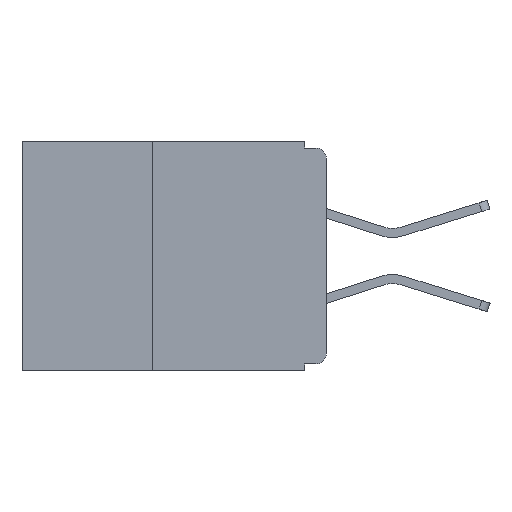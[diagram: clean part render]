
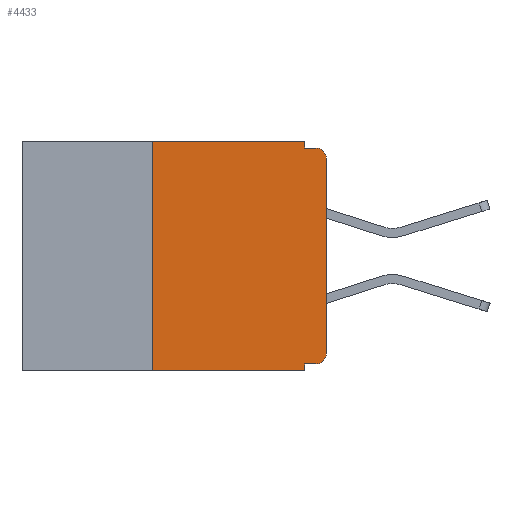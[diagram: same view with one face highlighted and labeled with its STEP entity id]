
A CAD part, left-side view. The second image highlights one B-rep face of the part: STEP entity #4433.
In plain terms, the highlighted planar face has unit normal (-1, 0, 0).
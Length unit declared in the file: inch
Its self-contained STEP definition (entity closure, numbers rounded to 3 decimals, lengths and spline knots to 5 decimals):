
#143 = DIRECTION ( 'NONE',  ( 0., 0., -1. ) ) ;
#241 = VERTEX_POINT ( 'NONE', #3242 ) ;
#295 = LINE ( 'NONE', #6987, #11551 ) ;
#338 = VERTEX_POINT ( 'NONE', #4104 ) ;
#356 = LINE ( 'NONE', #8640, #9029 ) ;
#531 = CIRCLE ( 'NONE', #8546, 0.015 ) ;
#587 = DIRECTION ( 'NONE',  ( 0., -1., 0. ) ) ;
#668 = CARTESIAN_POINT ( 'NONE',  ( 0., 0.031, -0.32 ) ) ;
#701 = CARTESIAN_POINT ( 'NONE',  ( 0., 0.031, 0. ) ) ;
#715 = EDGE_CURVE ( 'NONE', #6366, #241, #531, .T. ) ;
#730 = ORIENTED_EDGE ( 'NONE', *, *, #1172, .F. ) ;
#902 = EDGE_CURVE ( 'NONE', #9289, #8954, #10670, .T. ) ;
#1133 = EDGE_CURVE ( 'NONE', #241, #338, #356, .T. ) ;
#1172 = EDGE_CURVE ( 'NONE', #3067, #4759, #10904, .T. ) ;
#1413 = EDGE_CURVE ( 'NONE', #3067, #8878, #1812, .T. ) ;
#1451 = VECTOR ( 'NONE', #7285, 39.37008 ) ;
#1494 = VECTOR ( 'NONE', #143, 39.37008 ) ;
#1535 = DIRECTION ( 'NONE',  ( -1., 0., 0. ) ) ;
#1683 = EDGE_CURVE ( 'NONE', #10951, #8878, #11115, .T. ) ;
#1812 = LINE ( 'NONE', #2842, #6569 ) ;
#1942 = EDGE_CURVE ( 'NONE', #6366, #10951, #11325, .T. ) ;
#2098 = ORIENTED_EDGE ( 'NONE', *, *, #1942, .F. ) ;
#2403 = ORIENTED_EDGE ( 'NONE', *, *, #715, .T. ) ;
#2525 = EDGE_CURVE ( 'NONE', #4759, #9289, #295, .T. ) ;
#2842 = CARTESIAN_POINT ( 'NONE',  ( 0., 0.437, -0.33 ) ) ;
#3067 = VERTEX_POINT ( 'NONE', #10509 ) ;
#3071 = CARTESIAN_POINT ( 'NONE',  ( 0., 0.031, 0. ) ) ;
#3242 = CARTESIAN_POINT ( 'NONE',  ( 0., 0., -0.305 ) ) ;
#4104 = CARTESIAN_POINT ( 'NONE',  ( 0., 0., -0.025 ) ) ;
#4120 = VECTOR ( 'NONE', #11245, 39.37008 ) ;
#4205 = ORIENTED_EDGE ( 'NONE', *, *, #1413, .T. ) ;
#4405 = DIRECTION ( 'NONE',  ( 0., 1., 0. ) ) ;
#4433 = ADVANCED_FACE ( 'NONE', ( #6149 ), #10952, .F. ) ;
#4553 = CARTESIAN_POINT ( 'NONE',  ( 0., 0., -0.01 ) ) ;
#4743 = DIRECTION ( 'NONE',  ( 0., -1., 0. ) ) ;
#4759 = VERTEX_POINT ( 'NONE', #5955 ) ;
#4965 = CARTESIAN_POINT ( 'NONE',  ( 0., 0.015, -0.01 ) ) ;
#5347 = AXIS2_PLACEMENT_3D ( 'NONE', #7201, #1535, #8045 ) ;
#5384 = ORIENTED_EDGE ( 'NONE', *, *, #8906, .F. ) ;
#5557 = CARTESIAN_POINT ( 'NONE',  ( 0., 0.015, -0.32 ) ) ;
#5897 = EDGE_LOOP ( 'NONE', ( #9355, #11417, #5384, #7728, #9868, #730, #4205, #8853, #2098, #2403 ) ) ;
#5955 = CARTESIAN_POINT ( 'NONE',  ( 0., 0.25, 0. ) ) ;
#6149 = FACE_OUTER_BOUND ( 'NONE', #5897, .T. ) ;
#6366 = VERTEX_POINT ( 'NONE', #5557 ) ;
#6486 = LINE ( 'NONE', #4553, #10823 ) ;
#6569 = VECTOR ( 'NONE', #11216, 39.37008 ) ;
#6832 = VECTOR ( 'NONE', #4405, 39.37008 ) ;
#6900 = CARTESIAN_POINT ( 'NONE',  ( 0., 0.031, -0.33 ) ) ;
#6987 = CARTESIAN_POINT ( 'NONE',  ( 0., 0.437, 0. ) ) ;
#7201 = CARTESIAN_POINT ( 'NONE',  ( 0., 0.015, -0.025 ) ) ;
#7285 = DIRECTION ( 'NONE',  ( 0., 0., -1. ) ) ;
#7377 = EDGE_CURVE ( 'NONE', #338, #9231, #8599, .T. ) ;
#7728 = ORIENTED_EDGE ( 'NONE', *, *, #902, .F. ) ;
#7897 = AXIS2_PLACEMENT_3D ( 'NONE', #10851, #10834, #10822 ) ;
#8045 = DIRECTION ( 'NONE',  ( 0., 0., -1. ) ) ;
#8546 = AXIS2_PLACEMENT_3D ( 'NONE', #8711, #9264, #9254 ) ;
#8599 = CIRCLE ( 'NONE', #5347, 0.015 ) ;
#8640 = CARTESIAN_POINT ( 'NONE',  ( 0., 0., 0. ) ) ;
#8711 = CARTESIAN_POINT ( 'NONE',  ( 0., 0.015, -0.305 ) ) ;
#8853 = ORIENTED_EDGE ( 'NONE', *, *, #1683, .F. ) ;
#8878 = VERTEX_POINT ( 'NONE', #9696 ) ;
#8906 = EDGE_CURVE ( 'NONE', #8954, #9231, #6486, .T. ) ;
#8954 = VERTEX_POINT ( 'NONE', #11226 ) ;
#9029 = VECTOR ( 'NONE', #9837, 39.37008 ) ;
#9231 = VERTEX_POINT ( 'NONE', #4965 ) ;
#9254 = DIRECTION ( 'NONE',  ( 0., 0., -1. ) ) ;
#9264 = DIRECTION ( 'NONE',  ( -1., 0., 0. ) ) ;
#9289 = VERTEX_POINT ( 'NONE', #3071 ) ;
#9355 = ORIENTED_EDGE ( 'NONE', *, *, #1133, .T. ) ;
#9696 = CARTESIAN_POINT ( 'NONE',  ( 0., 0.031, -0.33 ) ) ;
#9837 = DIRECTION ( 'NONE',  ( 0., 0., 1. ) ) ;
#9868 = ORIENTED_EDGE ( 'NONE', *, *, #2525, .F. ) ;
#10189 = CARTESIAN_POINT ( 'NONE',  ( 0., 0.25, -0.33 ) ) ;
#10509 = CARTESIAN_POINT ( 'NONE',  ( 0., 0.25, -0.33 ) ) ;
#10668 = CARTESIAN_POINT ( 'NONE',  ( 0., 0., -0.32 ) ) ;
#10670 = LINE ( 'NONE', #701, #1494 ) ;
#10822 = DIRECTION ( 'NONE',  ( 0., 0., -1. ) ) ;
#10823 = VECTOR ( 'NONE', #587, 39.37008 ) ;
#10834 = DIRECTION ( 'NONE',  ( 1., 0., 0. ) ) ;
#10851 = CARTESIAN_POINT ( 'NONE',  ( 0., 0.437, 0. ) ) ;
#10904 = LINE ( 'NONE', #10189, #4120 ) ;
#10951 = VERTEX_POINT ( 'NONE', #668 ) ;
#10952 = PLANE ( 'NONE',  #7897 ) ;
#11115 = LINE ( 'NONE', #6900, #1451 ) ;
#11216 = DIRECTION ( 'NONE',  ( 0., -1., 0. ) ) ;
#11226 = CARTESIAN_POINT ( 'NONE',  ( 0., 0.031, -0.01 ) ) ;
#11245 = DIRECTION ( 'NONE',  ( 0., 0., 1. ) ) ;
#11325 = LINE ( 'NONE', #10668, #6832 ) ;
#11417 = ORIENTED_EDGE ( 'NONE', *, *, #7377, .T. ) ;
#11551 = VECTOR ( 'NONE', #4743, 39.37008 ) ;
